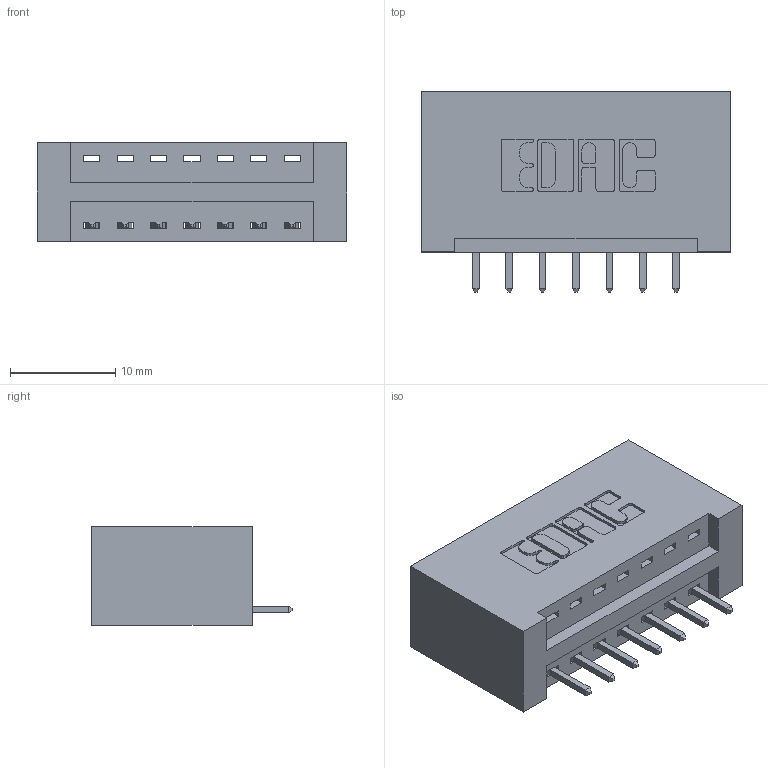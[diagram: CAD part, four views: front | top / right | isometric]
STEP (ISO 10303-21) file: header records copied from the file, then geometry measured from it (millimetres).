
FILE_DESCRIPTION (( 'STEP AP203' ), '1' );
FILE_NAME ('396-007-521-101.STEP', '2022-05-17T05:07:53', ( '' ), ( '' ), 'SwSTEP 2.0', 'SolidWorks 2020', '' );
FILE_SCHEMA (( 'CONFIG_CONTROL_DESIGN' ));
Length unit declared in the file: inch
Products named in the file (3): 346 Part_No Mounting Lugs; 396-007-521-101; 345-292-001_345-293-121
Assembly tree (8 placements, depth 2):
  396-007-521-101
    346 Part_No Mounting Lugs
    345-292-001_345-293-121  x7
Bounding box: 29.46 x 19.05 x 9.4 mm (x, y, z)
Volume: 3108.7 mm3; surface area: 3503.7 mm2
Topology: 8 solids, 8 shells, 520 faces, 1537 edges, 1014 vertices
Faces by surface type: plane 352, cylinder 168
Entity records: 8797 total; most frequent: CARTESIAN_POINT 1525, ORIENTED_EDGE 1466, DIRECTION 1383, EDGE_CURVE 733, VECTOR 581, LINE 581, VERTEX_POINT 486, AXIS2_PLACEMENT_3D 401
